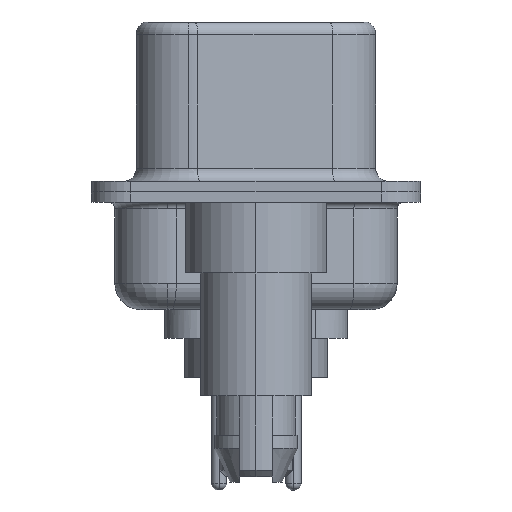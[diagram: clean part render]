
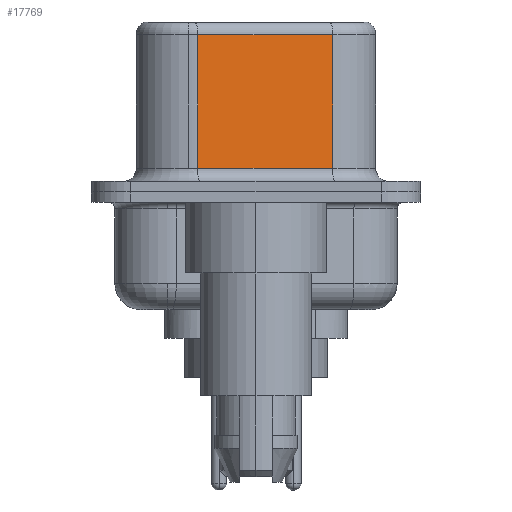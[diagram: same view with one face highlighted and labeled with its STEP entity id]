
A CAD part, left-side view. The second image highlights one B-rep face of the part: STEP entity #17769.
In plain terms, the highlighted planar face has unit normal (-0.985, -0.174, 0).
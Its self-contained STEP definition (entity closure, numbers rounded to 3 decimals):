
#384 = CARTESIAN_POINT ( 'NONE',  ( 3.675, 2.233, 6.52 ) ) ;
#507 = CARTESIAN_POINT ( 'NONE',  ( 3.675, 2.233, 0.9 ) ) ;
#524 = ORIENTED_EDGE ( 'NONE', *, *, #11435, .T. ) ;
#1158 = DIRECTION ( 'NONE',  ( -0.174, 0.985, 0. ) ) ;
#1485 = ORIENTED_EDGE ( 'NONE', *, *, #6784, .T. ) ;
#2310 = VERTEX_POINT ( 'NONE', #8733 ) ;
#2763 = EDGE_CURVE ( 'NONE', #10605, #2310, #15093, .T. ) ;
#4065 = AXIS2_PLACEMENT_3D ( 'NONE', #7595, #7666, #18629 ) ;
#4446 = VERTEX_POINT ( 'NONE', #507 ) ;
#4530 = VECTOR ( 'NONE', #19052, 1000. ) ;
#5321 = DIRECTION ( 'NONE',  ( 0.174, -0.985, 0. ) ) ;
#6459 = DIRECTION ( 'NONE',  ( 0., 0., -1. ) ) ;
#6676 = VERTEX_POINT ( 'NONE', #17091 ) ;
#6784 = EDGE_CURVE ( 'NONE', #2310, #4446, #7308, .T. ) ;
#6809 = FACE_OUTER_BOUND ( 'NONE', #17596, .T. ) ;
#7012 = ORIENTED_EDGE ( 'NONE', *, *, #14191, .F. ) ;
#7308 = LINE ( 'NONE', #384, #15154 ) ;
#7595 = CARTESIAN_POINT ( 'NONE',  ( 4.585, -2.927, 6.52 ) ) ;
#7666 = DIRECTION ( 'NONE',  ( 0.985, 0.174, 0. ) ) ;
#8090 = CARTESIAN_POINT ( 'NONE',  ( 4.585, -2.927, 6.52 ) ) ;
#8733 = CARTESIAN_POINT ( 'NONE',  ( 3.675, 2.233, 6.02 ) ) ;
#10605 = VERTEX_POINT ( 'NONE', #10881 ) ;
#10881 = CARTESIAN_POINT ( 'NONE',  ( 4.585, -2.927, 6.02 ) ) ;
#11020 = CARTESIAN_POINT ( 'NONE',  ( 4.585, -2.927, 0.9 ) ) ;
#11363 = VECTOR ( 'NONE', #5321, 1000. ) ;
#11435 = EDGE_CURVE ( 'NONE', #4446, #6676, #15498, .T. ) ;
#12813 = LINE ( 'NONE', #8090, #4530 ) ;
#13718 = ORIENTED_EDGE ( 'NONE', *, *, #2763, .T. ) ;
#13885 = PLANE ( 'NONE',  #4065 ) ;
#14191 = EDGE_CURVE ( 'NONE', #10605, #6676, #12813, .T. ) ;
#15093 = LINE ( 'NONE', #18754, #19797 ) ;
#15154 = VECTOR ( 'NONE', #6459, 1000. ) ;
#15498 = LINE ( 'NONE', #11020, #11363 ) ;
#17091 = CARTESIAN_POINT ( 'NONE',  ( 4.585, -2.927, 0.9 ) ) ;
#17596 = EDGE_LOOP ( 'NONE', ( #7012, #13718, #1485, #524 ) ) ;
#17769 = ADVANCED_FACE ( 'NONE', ( #6809 ), #13885, .F. ) ;
#18629 = DIRECTION ( 'NONE',  ( -0.174, 0.985, 0. ) ) ;
#18754 = CARTESIAN_POINT ( 'NONE',  ( 4.585, -2.927, 6.02 ) ) ;
#19052 = DIRECTION ( 'NONE',  ( 0., 0., -1. ) ) ;
#19797 = VECTOR ( 'NONE', #1158, 1000. ) ;
